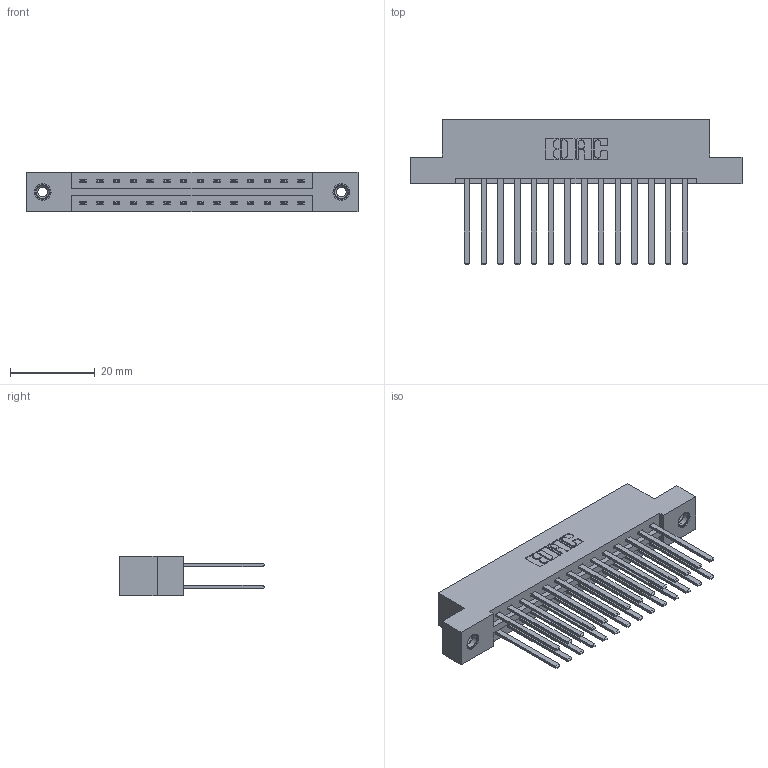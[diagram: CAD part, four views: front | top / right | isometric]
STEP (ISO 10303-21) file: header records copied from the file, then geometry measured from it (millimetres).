
FILE_DESCRIPTION (( 'STEP AP203' ), '1' );
FILE_NAME ('387-028-544-208.STEP', '2019-10-16T22:28:14', ( '' ), ( '' ), 'SwSTEP 2.0', 'SolidWorks 2016', '' );
FILE_SCHEMA (( 'CONFIG_CONTROL_DESIGN' ));
Length unit declared in the file: inch
Products named in the file (4): 337 Part_Flush Mounting Lugs - 0.156 Dia-TI; 345-250-001_345-250-003-102; 387-028-544-208; 345-292-001_345-293-144
Assembly tree (31 placements, depth 2):
  387-028-544-208
    337 Part_Flush Mounting Lugs - 0.156 Dia-TI
    345-292-001_345-293-144  x28
    345-250-001_345-250-003-102  x2
Bounding box: 78.49 x 34.3 x 9.4 mm (x, y, z)
Volume: 8284.8 mm3; surface area: 10400.1 mm2
Topology: 31 solids, 31 shells, 1518 faces, 4451 edges, 2922 vertices
Faces by surface type: plane 1054, cylinder 448, cone 12, torus 4
Entity records: 15478 total; most frequent: CARTESIAN_POINT 2609, ORIENTED_EDGE 2538, DIRECTION 2299, EDGE_CURVE 1269, VECTOR 1125, LINE 1125, VERTEX_POINT 840, AXIS2_PLACEMENT_3D 587
